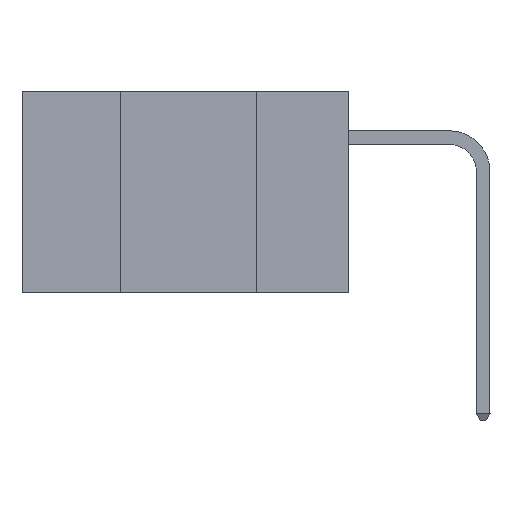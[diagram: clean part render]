
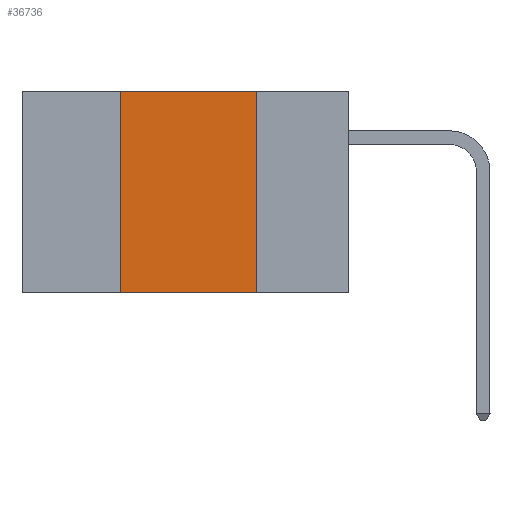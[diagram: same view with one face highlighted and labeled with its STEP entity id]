
A CAD part, left-side view. The second image highlights one B-rep face of the part: STEP entity #36736.
In plain terms, the highlighted planar face has unit normal (-1, 0, 0).
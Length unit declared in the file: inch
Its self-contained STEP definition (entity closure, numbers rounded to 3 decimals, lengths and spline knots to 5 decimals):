
#94 = VERTEX_POINT ( 'NONE', #40820 ) ;
#146 = VERTEX_POINT ( 'NONE', #35248 ) ;
#339 = EDGE_LOOP ( 'NONE', ( #20876, #22180, #16052, #28116 ) ) ;
#1997 = CARTESIAN_POINT ( 'NONE',  ( 0., 0.42, -0.37 ) ) ;
#2046 = CARTESIAN_POINT ( 'NONE',  ( 0., 0.6, -0.37 ) ) ;
#9271 = DIRECTION ( 'NONE',  ( 0., -1., 0. ) ) ;
#9438 = VECTOR ( 'NONE', #17977, 39.37008 ) ;
#10651 = VECTOR ( 'NONE', #9271, 39.37008 ) ;
#11205 = CARTESIAN_POINT ( 'NONE',  ( 0., 0.42, 0. ) ) ;
#11991 = EDGE_CURVE ( 'NONE', #146, #94, #34592, .T. ) ;
#14124 = CARTESIAN_POINT ( 'NONE',  ( 0., 0.42, 0. ) ) ;
#14226 = PLANE ( 'NONE',  #39630 ) ;
#14804 = LINE ( 'NONE', #27817, #10651 ) ;
#16052 = ORIENTED_EDGE ( 'NONE', *, *, #21503, .F. ) ;
#17977 = DIRECTION ( 'NONE',  ( 0., 0., -1. ) ) ;
#19298 = LINE ( 'NONE', #2046, #28396 ) ;
#20431 = FACE_OUTER_BOUND ( 'NONE', #339, .T. ) ;
#20876 = ORIENTED_EDGE ( 'NONE', *, *, #11991, .F. ) ;
#21503 = EDGE_CURVE ( 'NONE', #38729, #24015, #30331, .T. ) ;
#22180 = ORIENTED_EDGE ( 'NONE', *, *, #28903, .F. ) ;
#24015 = VERTEX_POINT ( 'NONE', #11205 ) ;
#25232 = CARTESIAN_POINT ( 'NONE',  ( 0., 0.17, 0. ) ) ;
#27010 = DIRECTION ( 'NONE',  ( 1., 0., 0. ) ) ;
#27235 = CARTESIAN_POINT ( 'NONE',  ( 0., 0.6, 0. ) ) ;
#27548 = DIRECTION ( 'NONE',  ( 0., 0., 1. ) ) ;
#27817 = CARTESIAN_POINT ( 'NONE',  ( 0., 0.6, 0. ) ) ;
#28050 = DIRECTION ( 'NONE',  ( 0., -1., 0. ) ) ;
#28116 = ORIENTED_EDGE ( 'NONE', *, *, #29753, .T. ) ;
#28396 = VECTOR ( 'NONE', #28050, 39.37008 ) ;
#28903 = EDGE_CURVE ( 'NONE', #24015, #146, #14804, .T. ) ;
#29753 = EDGE_CURVE ( 'NONE', #38729, #94, #19298, .T. ) ;
#30331 = LINE ( 'NONE', #14124, #30470 ) ;
#30470 = VECTOR ( 'NONE', #27548, 39.37008 ) ;
#30860 = DIRECTION ( 'NONE',  ( 0., 0., -1. ) ) ;
#34592 = LINE ( 'NONE', #25232, #9438 ) ;
#35248 = CARTESIAN_POINT ( 'NONE',  ( 0., 0.17, 0. ) ) ;
#36736 = ADVANCED_FACE ( 'NONE', ( #20431 ), #14226, .F. ) ;
#38729 = VERTEX_POINT ( 'NONE', #1997 ) ;
#39630 = AXIS2_PLACEMENT_3D ( 'NONE', #27235, #27010, #30860 ) ;
#40820 = CARTESIAN_POINT ( 'NONE',  ( 0., 0.17, -0.37 ) ) ;
